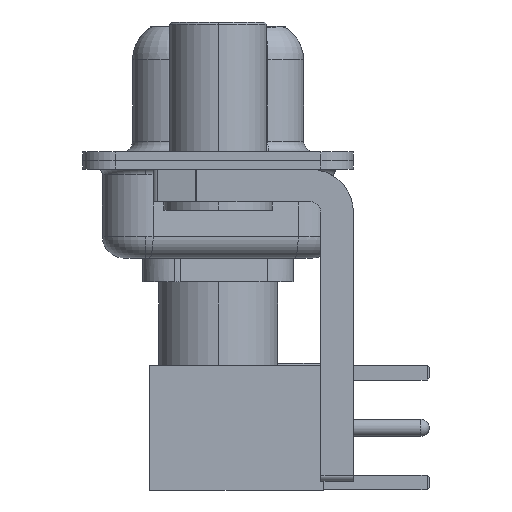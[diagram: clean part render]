
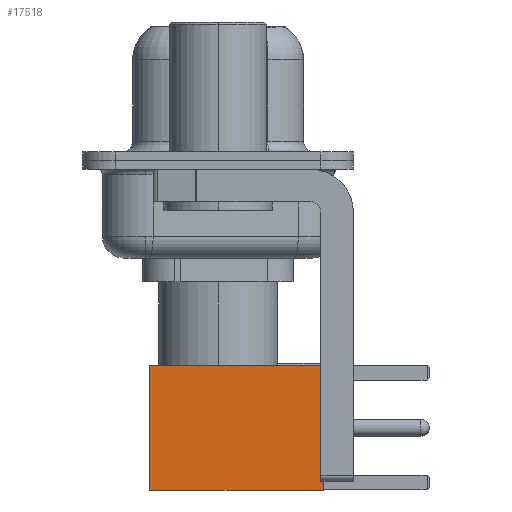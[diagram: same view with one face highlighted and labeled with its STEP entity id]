
A CAD part, left-side view. The second image highlights one B-rep face of the part: STEP entity #17518.
In plain terms, the highlighted face is planar.
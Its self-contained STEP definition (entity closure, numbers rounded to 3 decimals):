
#390 = LINE ( 'NONE', #2429, #21913 ) ;
#1379 = EDGE_LOOP ( 'NONE', ( #18152, #13793, #8089, #23611 ) ) ;
#1807 = PLANE ( 'NONE',  #26155 ) ;
#2429 = CARTESIAN_POINT ( 'NONE',  ( 2.875, 2.875, 0. ) ) ;
#3453 = VECTOR ( 'NONE', #10673, 1000. ) ;
#3597 = LINE ( 'NONE', #23896, #14491 ) ;
#3730 = DIRECTION ( 'NONE',  ( -1., 0., 0. ) ) ;
#4520 = CARTESIAN_POINT ( 'NONE',  ( 0., 2.875, 8. ) ) ;
#4828 = EDGE_CURVE ( 'NONE', #13479, #22706, #16688, .T. ) ;
#5169 = CARTESIAN_POINT ( 'NONE',  ( -2.875, 2.875, 8. ) ) ;
#5684 = EDGE_CURVE ( 'NONE', #9786, #25053, #3597, .T. ) ;
#6799 = DIRECTION ( 'NONE',  ( 0., 0., -1. ) ) ;
#8089 = ORIENTED_EDGE ( 'NONE', *, *, #25560, .F. ) ;
#8117 = DIRECTION ( 'NONE',  ( 0., 0., -1. ) ) ;
#9786 = VERTEX_POINT ( 'NONE', #14329 ) ;
#10070 = CARTESIAN_POINT ( 'NONE',  ( -2.875, 2.875, 0. ) ) ;
#10673 = DIRECTION ( 'NONE',  ( -1., 0., 0. ) ) ;
#11788 = DIRECTION ( 'NONE',  ( 0., 1., 0. ) ) ;
#13479 = VERTEX_POINT ( 'NONE', #20893 ) ;
#13793 = ORIENTED_EDGE ( 'NONE', *, *, #5684, .T. ) ;
#14329 = CARTESIAN_POINT ( 'NONE',  ( 2.875, 2.875, 0. ) ) ;
#14375 = DIRECTION ( 'NONE',  ( 0., 0., 1. ) ) ;
#14491 = VECTOR ( 'NONE', #3730, 1000. ) ;
#16688 = LINE ( 'NONE', #4520, #3453 ) ;
#17518 = ADVANCED_FACE ( 'NONE', ( #26677 ), #1807, .T. ) ;
#18152 = ORIENTED_EDGE ( 'NONE', *, *, #19686, .T. ) ;
#19686 = EDGE_CURVE ( 'NONE', #13479, #9786, #390, .T. ) ;
#19908 = VECTOR ( 'NONE', #8117, 1000. ) ;
#20442 = LINE ( 'NONE', #26835, #19908 ) ;
#20893 = CARTESIAN_POINT ( 'NONE',  ( 2.875, 2.875, 8. ) ) ;
#21913 = VECTOR ( 'NONE', #6799, 1000. ) ;
#22706 = VERTEX_POINT ( 'NONE', #5169 ) ;
#22885 = CARTESIAN_POINT ( 'NONE',  ( 2.875, 2.875, 0. ) ) ;
#23611 = ORIENTED_EDGE ( 'NONE', *, *, #4828, .F. ) ;
#23896 = CARTESIAN_POINT ( 'NONE',  ( 0., 2.875, 0. ) ) ;
#25053 = VERTEX_POINT ( 'NONE', #10070 ) ;
#25560 = EDGE_CURVE ( 'NONE', #22706, #25053, #20442, .T. ) ;
#26155 = AXIS2_PLACEMENT_3D ( 'NONE', #22885, #11788, #14375 ) ;
#26677 = FACE_OUTER_BOUND ( 'NONE', #1379, .T. ) ;
#26835 = CARTESIAN_POINT ( 'NONE',  ( -2.875, 2.875, 0. ) ) ;
